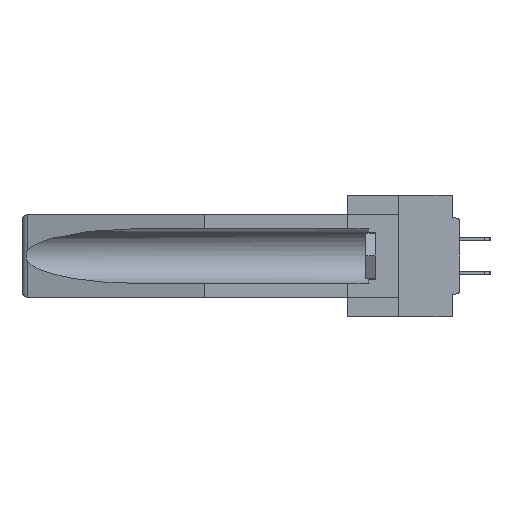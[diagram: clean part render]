
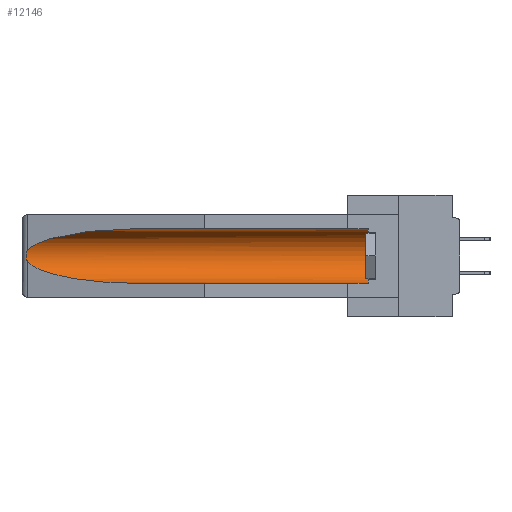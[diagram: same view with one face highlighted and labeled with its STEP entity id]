
A CAD part, left-side view. The second image highlights one B-rep face of the part: STEP entity #12146.
In plain terms, the highlighted cylindrical face has radius 2.857 mm (diameter 5.715 mm), a partial arc.
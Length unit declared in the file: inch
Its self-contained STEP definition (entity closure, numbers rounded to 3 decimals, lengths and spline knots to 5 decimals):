
#108 = CARTESIAN_POINT ( 'NONE',  ( 0.26597, 1.52961, -0.15275 ) ) ;
#804 = VECTOR ( 'NONE', #30558, 39.37008 ) ;
#1579 = DIRECTION ( 'NONE',  ( 0., 1., 0. ) ) ;
#2778 = CARTESIAN_POINT ( 'NONE',  ( 0.2675, 1.53308, -0.16763 ) ) ;
#3706 = EDGE_CURVE ( 'NONE', #27950, #4436, #6659, .T. ) ;
#3792 = CARTESIAN_POINT ( 'NONE',  ( 0.155, -0.30754, -0.1715 ) ) ;
#4030 = DIRECTION ( 'NONE',  ( 0., 1., 0. ) ) ;
#4057 = CARTESIAN_POINT ( 'NONE',  ( 0.155, -0.30754, -0.059 ) ) ;
#4436 = VERTEX_POINT ( 'NONE', #15499 ) ;
#4893 = VECTOR ( 'NONE', #1579, 39.37008 ) ;
#4945 = AXIS2_PLACEMENT_3D ( 'NONE', #11118, #35967, #14071 ) ;
#5053 = EDGE_CURVE ( 'NONE', #26181, #27950, #26648, .T. ) ;
#5185 = EDGE_LOOP ( 'NONE', ( #15767, #32414, #35944, #11549, #16128, #9667 ) ) ;
#5716 = CARTESIAN_POINT ( 'NONE',  ( 0.25451, 1.48313, -0.09465 ) ) ;
#6659 = LINE ( 'NONE', #4057, #4893 ) ;
#8136 = CYLINDRICAL_SURFACE ( 'NONE', #28703, 0.1125 ) ;
#9313 = DIRECTION ( 'NONE',  ( 0., 0., 1. ) ) ;
#9431 = CARTESIAN_POINT ( 'NONE',  ( 0.26537, 1.52718, -0.19328 ) ) ;
#9667 = ORIENTED_EDGE ( 'NONE', *, *, #3706, .T. ) ;
#10168 = CARTESIAN_POINT ( 'NONE',  ( 0.155, 1.07973, -0.284 ) ) ;
#10301 = FACE_OUTER_BOUND ( 'NONE', #5185, .T. ) ;
#10964 = CARTESIAN_POINT ( 'NONE',  ( 0.155, -0.30754, -0.284 ) ) ;
#10989 = CARTESIAN_POINT ( 'NONE',  ( 0.2675, 1.53308, -0.17534 ) ) ;
#11118 = CARTESIAN_POINT ( 'NONE',  ( 0.155, 0.126, -0.1715 ) ) ;
#11549 = ORIENTED_EDGE ( 'NONE', *, *, #26341, .F. ) ;
#11892 = CARTESIAN_POINT ( 'NONE',  ( 0.26537, 1.52718, -0.19328 ) ) ;
#12146 = ADVANCED_FACE ( 'NONE', ( #10301 ), #8136, .F. ) ;
#12245 = VERTEX_POINT ( 'NONE', #9431 ) ;
#14071 = DIRECTION ( 'NONE',  ( 0., 0., 1. ) ) ;
#15002 = CARTESIAN_POINT ( 'NONE',  ( 0.155, 0.126, -0.059 ) ) ;
#15499 = CARTESIAN_POINT ( 'NONE',  ( 0.155, 1.07973, -0.059 ) ) ;
#15767 = ORIENTED_EDGE ( 'NONE', *, *, #32661, .T. ) ;
#16128 = ORIENTED_EDGE ( 'NONE', *, *, #5053, .T. ) ;
#16388 = EDGE_CURVE ( 'NONE', #12245, #20992, #26690, .T. ) ;
#16857 = CARTESIAN_POINT ( 'NONE',  ( 0.26537, 1.52718, -0.14972 ) ) ;
#18002 = EDGE_CURVE ( 'NONE', #27375, #12245, #20224, .T. ) ;
#18634 =( BOUNDED_CURVE ( )  B_SPLINE_CURVE ( 3, ( #33630, #19898, #5716, #28079 ),
 .UNSPECIFIED., .F., .F. ) 
 B_SPLINE_CURVE_WITH_KNOTS ( ( 4, 4 ),
 ( 4.71239, 6.08839 ),
 .UNSPECIFIED. ) 
 CURVE ( )  GEOMETRIC_REPRESENTATION_ITEM ( )  RATIONAL_B_SPLINE_CURVE ( ( 1., 0.848, 0.848, 1. ) ) 
 REPRESENTATION_ITEM ( '' )  );
#19898 = CARTESIAN_POINT ( 'NONE',  ( 0.21114, 1.30732, -0.059 ) ) ;
#20224 = B_SPLINE_CURVE_WITH_KNOTS ( 'NONE', 3,
 ( #16857, #108, #25177, #33408, #2778, #10989, #22116, #27612, #22352, #27975 ),
 .UNSPECIFIED., .F., .F.,
 ( 4, 2, 2, 2, 4 ),
 ( 0., 0.00029, 0.00058, 0.00087, 0.00117 ),
 .UNSPECIFIED. ) ;
#20539 = CARTESIAN_POINT ( 'NONE',  ( 0.25451, 1.48313, -0.24835 ) ) ;
#20936 = LINE ( 'NONE', #10964, #804 ) ;
#20992 = VERTEX_POINT ( 'NONE', #10168 ) ;
#22116 = CARTESIAN_POINT ( 'NONE',  ( 0.2673, 1.53269, -0.17917 ) ) ;
#22352 = CARTESIAN_POINT ( 'NONE',  ( 0.26597, 1.5296, -0.19026 ) ) ;
#25177 = CARTESIAN_POINT ( 'NONE',  ( 0.26654, 1.53092, -0.15636 ) ) ;
#26181 = VERTEX_POINT ( 'NONE', #35363 ) ;
#26341 = EDGE_CURVE ( 'NONE', #26181, #20992, #20936, .T. ) ;
#26648 = CIRCLE ( 'NONE', #4945, 0.1125 ) ;
#26690 =( BOUNDED_CURVE ( )  B_SPLINE_CURVE ( 3, ( #11892, #20539, #34307, #28641 ),
 .UNSPECIFIED., .F., .F. ) 
 B_SPLINE_CURVE_WITH_KNOTS ( ( 4, 4 ),
 ( 0.1948, 1.5708 ),
 .UNSPECIFIED. ) 
 CURVE ( )  GEOMETRIC_REPRESENTATION_ITEM ( )  RATIONAL_B_SPLINE_CURVE ( ( 1., 0.848, 0.848, 1. ) ) 
 REPRESENTATION_ITEM ( '' )  );
#27375 = VERTEX_POINT ( 'NONE', #29868 ) ;
#27612 = CARTESIAN_POINT ( 'NONE',  ( 0.26655, 1.53094, -0.18657 ) ) ;
#27950 = VERTEX_POINT ( 'NONE', #15002 ) ;
#27975 = CARTESIAN_POINT ( 'NONE',  ( 0.26537, 1.52718, -0.19328 ) ) ;
#28079 = CARTESIAN_POINT ( 'NONE',  ( 0.26537, 1.52718, -0.14972 ) ) ;
#28641 = CARTESIAN_POINT ( 'NONE',  ( 0.155, 1.07973, -0.284 ) ) ;
#28703 = AXIS2_PLACEMENT_3D ( 'NONE', #3792, #4030, #9313 ) ;
#29868 = CARTESIAN_POINT ( 'NONE',  ( 0.26537, 1.52718, -0.14972 ) ) ;
#30558 = DIRECTION ( 'NONE',  ( 0., 1., 0. ) ) ;
#32414 = ORIENTED_EDGE ( 'NONE', *, *, #18002, .T. ) ;
#32661 = EDGE_CURVE ( 'NONE', #4436, #27375, #18634, .T. ) ;
#33408 = CARTESIAN_POINT ( 'NONE',  ( 0.2673, 1.5327, -0.16383 ) ) ;
#33630 = CARTESIAN_POINT ( 'NONE',  ( 0.155, 1.07973, -0.059 ) ) ;
#34307 = CARTESIAN_POINT ( 'NONE',  ( 0.21114, 1.30732, -0.284 ) ) ;
#35363 = CARTESIAN_POINT ( 'NONE',  ( 0.155, 0.126, -0.284 ) ) ;
#35944 = ORIENTED_EDGE ( 'NONE', *, *, #16388, .T. ) ;
#35967 = DIRECTION ( 'NONE',  ( 0., -1., 0. ) ) ;
